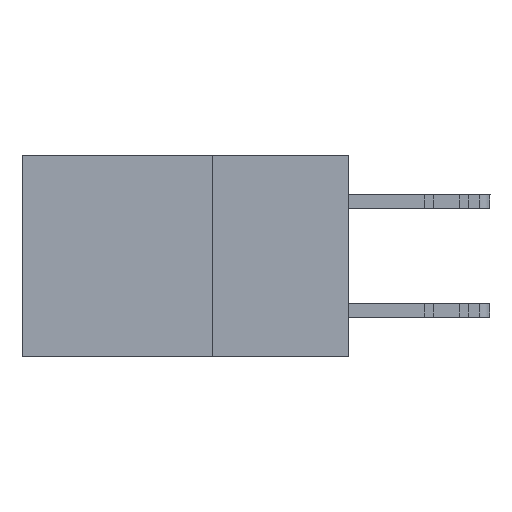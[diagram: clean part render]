
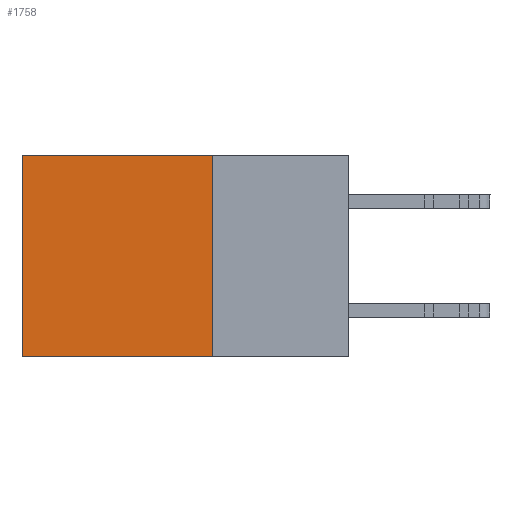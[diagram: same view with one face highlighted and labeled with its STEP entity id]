
A CAD part, left-side view. The second image highlights one B-rep face of the part: STEP entity #1758.
In plain terms, the highlighted planar face has unit normal (-1, 0, 0).
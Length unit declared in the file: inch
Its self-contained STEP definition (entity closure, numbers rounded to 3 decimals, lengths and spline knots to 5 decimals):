
#1369 = FACE_OUTER_BOUND ( 'NONE', #30641, .T. ) ;
#1515 = EDGE_CURVE ( 'NONE', #2091, #12954, #7229, .T. ) ;
#1758 = ADVANCED_FACE ( 'NONE', ( #1369 ), #29413, .F. ) ;
#2091 = VERTEX_POINT ( 'NONE', #10575 ) ;
#2353 = CARTESIAN_POINT ( 'NONE',  ( 0.298, 0.6, -0.37 ) ) ;
#2897 = CARTESIAN_POINT ( 'NONE',  ( 0.298, 0.25, 0. ) ) ;
#3262 = DIRECTION ( 'NONE',  ( 1., 0., 0. ) ) ;
#4578 = ORIENTED_EDGE ( 'NONE', *, *, #7336, .T. ) ;
#6539 = AXIS2_PLACEMENT_3D ( 'NONE', #19010, #3262, #24295 ) ;
#7050 = DIRECTION ( 'NONE',  ( 0., 1., 0. ) ) ;
#7229 = LINE ( 'NONE', #9612, #19092 ) ;
#7336 = EDGE_CURVE ( 'NONE', #14474, #31745, #21353, .T. ) ;
#9009 = ORIENTED_EDGE ( 'NONE', *, *, #15100, .F. ) ;
#9124 = VECTOR ( 'NONE', #30639, 39.37008 ) ;
#9612 = CARTESIAN_POINT ( 'NONE',  ( 0.298, 0.25, -0.37 ) ) ;
#10575 = CARTESIAN_POINT ( 'NONE',  ( 0.298, 0.25, -0.37 ) ) ;
#11110 = CARTESIAN_POINT ( 'NONE',  ( 0.298, 0.25, 0. ) ) ;
#11687 = CARTESIAN_POINT ( 'NONE',  ( 0.298, 0.6, 0. ) ) ;
#12529 = EDGE_CURVE ( 'NONE', #31745, #12954, #17331, .T. ) ;
#12954 = VERTEX_POINT ( 'NONE', #2353 ) ;
#14474 = VERTEX_POINT ( 'NONE', #11110 ) ;
#15100 = EDGE_CURVE ( 'NONE', #14474, #2091, #33157, .T. ) ;
#17331 = LINE ( 'NONE', #11687, #27336 ) ;
#19010 = CARTESIAN_POINT ( 'NONE',  ( 0.298, 0.25, 0. ) ) ;
#19092 = VECTOR ( 'NONE', #7050, 39.37008 ) ;
#20085 = DIRECTION ( 'NONE',  ( 0., 0., -1. ) ) ;
#21353 = LINE ( 'NONE', #2897, #21452 ) ;
#21452 = VECTOR ( 'NONE', #31890, 39.37008 ) ;
#22138 = ORIENTED_EDGE ( 'NONE', *, *, #1515, .F. ) ;
#23662 = CARTESIAN_POINT ( 'NONE',  ( 0.298, 0.6, 0. ) ) ;
#24295 = DIRECTION ( 'NONE',  ( 0., 0., -1. ) ) ;
#26772 = ORIENTED_EDGE ( 'NONE', *, *, #12529, .T. ) ;
#27336 = VECTOR ( 'NONE', #20085, 39.37008 ) ;
#27594 = CARTESIAN_POINT ( 'NONE',  ( 0.298, 0.25, 0. ) ) ;
#29413 = PLANE ( 'NONE',  #6539 ) ;
#30639 = DIRECTION ( 'NONE',  ( 0., 0., -1. ) ) ;
#30641 = EDGE_LOOP ( 'NONE', ( #26772, #22138, #9009, #4578 ) ) ;
#31745 = VERTEX_POINT ( 'NONE', #23662 ) ;
#31890 = DIRECTION ( 'NONE',  ( 0., 1., 0. ) ) ;
#33157 = LINE ( 'NONE', #27594, #9124 ) ;
